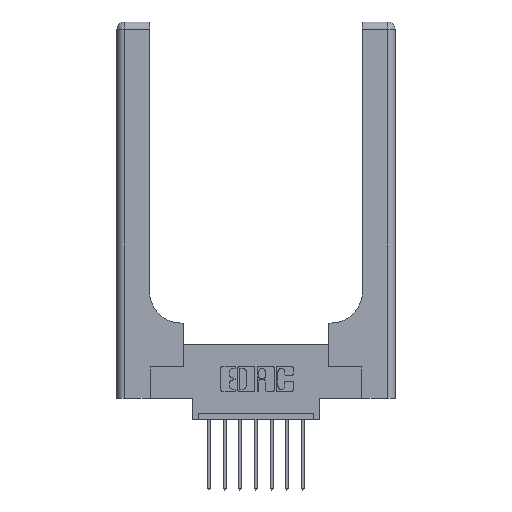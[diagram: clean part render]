
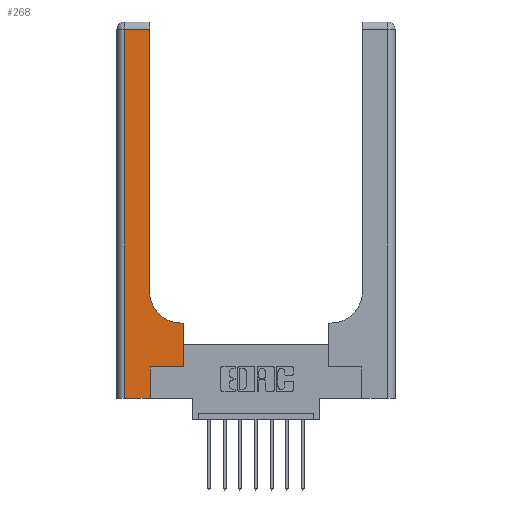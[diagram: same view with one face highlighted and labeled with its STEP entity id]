
A CAD part, top view. The second image highlights one B-rep face of the part: STEP entity #268.
In plain terms, the highlighted planar face has unit normal (0, 0, 1).
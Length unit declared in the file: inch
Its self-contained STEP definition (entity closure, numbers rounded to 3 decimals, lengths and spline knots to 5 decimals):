
#268 = ADVANCED_FACE ( 'NONE', ( #9677 ), #9599, .F. ) ;
#281 = VECTOR ( 'NONE', #3276, 39.37008 ) ;
#473 = EDGE_LOOP ( 'NONE', ( #7348, #3690, #8259, #9559, #8176, #2002, #1999, #13396, #4177 ) ) ;
#953 = LINE ( 'NONE', #8980, #11258 ) ;
#1074 = EDGE_CURVE ( 'NONE', #9855, #10278, #6020, .T. ) ;
#1240 = EDGE_CURVE ( 'NONE', #3831, #9855, #10203, .T. ) ;
#1338 = CARTESIAN_POINT ( 'NONE',  ( 0.528, 0.6, 0.37 ) ) ;
#1574 = LINE ( 'NONE', #5980, #10350 ) ;
#1582 = CARTESIAN_POINT ( 'NONE',  ( 0., 2.94, 0.37 ) ) ;
#1621 = DIRECTION ( 'NONE',  ( 1., 0., 0. ) ) ;
#1999 = ORIENTED_EDGE ( 'NONE', *, *, #14605, .T. ) ;
#2002 = ORIENTED_EDGE ( 'NONE', *, *, #8616, .T. ) ;
#2029 = CARTESIAN_POINT ( 'NONE',  ( 0.26, 0.6, 0.37 ) ) ;
#2476 = CARTESIAN_POINT ( 'NONE',  ( 0.26, 3., 0.37 ) ) ;
#2535 = DIRECTION ( 'NONE',  ( -1., 0., 0. ) ) ;
#2657 = CARTESIAN_POINT ( 'NONE',  ( 0.06, 0., 0.37 ) ) ;
#3129 = DIRECTION ( 'NONE',  ( 1., 0., 0. ) ) ;
#3276 = DIRECTION ( 'NONE',  ( -1., 0., 0. ) ) ;
#3508 = EDGE_CURVE ( 'NONE', #3846, #7573, #11775, .T. ) ;
#3520 = DIRECTION ( 'NONE',  ( 0., 0., -1. ) ) ;
#3690 = ORIENTED_EDGE ( 'NONE', *, *, #3508, .T. ) ;
#3748 = CARTESIAN_POINT ( 'NONE',  ( 0.06, 3., 0.37 ) ) ;
#3753 = VERTEX_POINT ( 'NONE', #8074 ) ;
#3831 = VERTEX_POINT ( 'NONE', #1338 ) ;
#3846 = VERTEX_POINT ( 'NONE', #7935 ) ;
#3858 = VECTOR ( 'NONE', #3129, 39.37008 ) ;
#3957 = CARTESIAN_POINT ( 'NONE',  ( 0., 3., 0.37 ) ) ;
#3981 = LINE ( 'NONE', #8408, #12728 ) ;
#4177 = ORIENTED_EDGE ( 'NONE', *, *, #1074, .T. ) ;
#4865 = LINE ( 'NONE', #2476, #13954 ) ;
#5476 = CARTESIAN_POINT ( 'NONE',  ( 0.265, 0., 0.37 ) ) ;
#5980 = CARTESIAN_POINT ( 'NONE',  ( 0.528, 0.25, 0.37 ) ) ;
#6020 = CIRCLE ( 'NONE', #10579, 0.25 ) ;
#6191 = EDGE_CURVE ( 'NONE', #7573, #10110, #14022, .T. ) ;
#7010 = EDGE_CURVE ( 'NONE', #13799, #3753, #3981, .T. ) ;
#7271 = DIRECTION ( 'NONE',  ( 0., 1., 0. ) ) ;
#7348 = ORIENTED_EDGE ( 'NONE', *, *, #8216, .T. ) ;
#7573 = VERTEX_POINT ( 'NONE', #13841 ) ;
#7856 = LINE ( 'NONE', #8767, #3858 ) ;
#7935 = CARTESIAN_POINT ( 'NONE',  ( 0.26, 2.94, 0.37 ) ) ;
#8074 = CARTESIAN_POINT ( 'NONE',  ( 0.265, 0.25, 0.37 ) ) ;
#8092 = DIRECTION ( 'NONE',  ( 1., 0., 0. ) ) ;
#8176 = ORIENTED_EDGE ( 'NONE', *, *, #7010, .T. ) ;
#8216 = EDGE_CURVE ( 'NONE', #10278, #3846, #4865, .T. ) ;
#8259 = ORIENTED_EDGE ( 'NONE', *, *, #6191, .T. ) ;
#8408 = CARTESIAN_POINT ( 'NONE',  ( 0.265, 0., 0.37 ) ) ;
#8616 = EDGE_CURVE ( 'NONE', #3753, #13579, #7856, .T. ) ;
#8767 = CARTESIAN_POINT ( 'NONE',  ( 0.265, 0.25, 0.37 ) ) ;
#8980 = CARTESIAN_POINT ( 'NONE',  ( 0., 0., 0.37 ) ) ;
#9240 = CARTESIAN_POINT ( 'NONE',  ( 0.51, 0.85, 0.37 ) ) ;
#9559 = ORIENTED_EDGE ( 'NONE', *, *, #10294, .T. ) ;
#9599 = PLANE ( 'NONE',  #14229 ) ;
#9677 = FACE_OUTER_BOUND ( 'NONE', #473, .T. ) ;
#9855 = VERTEX_POINT ( 'NONE', #10279 ) ;
#10110 = VERTEX_POINT ( 'NONE', #2657 ) ;
#10203 = LINE ( 'NONE', #2029, #281 ) ;
#10278 = VERTEX_POINT ( 'NONE', #10400 ) ;
#10279 = CARTESIAN_POINT ( 'NONE',  ( 0.51, 0.6, 0.37 ) ) ;
#10294 = EDGE_CURVE ( 'NONE', #10110, #13799, #953, .T. ) ;
#10350 = VECTOR ( 'NONE', #7271, 39.37008 ) ;
#10400 = CARTESIAN_POINT ( 'NONE',  ( 0.26, 0.85, 0.37 ) ) ;
#10579 = AXIS2_PLACEMENT_3D ( 'NONE', #9240, #3520, #8092 ) ;
#10660 = DIRECTION ( 'NONE',  ( -1., 0., 0. ) ) ;
#10769 = VECTOR ( 'NONE', #10660, 39.37008 ) ;
#11258 = VECTOR ( 'NONE', #1621, 39.37008 ) ;
#11775 = LINE ( 'NONE', #1582, #10769 ) ;
#11856 = DIRECTION ( 'NONE',  ( 0., 1., 0. ) ) ;
#12728 = VECTOR ( 'NONE', #11856, 39.37008 ) ;
#12757 = CARTESIAN_POINT ( 'NONE',  ( 0.528, 0.25, 0.37 ) ) ;
#12887 = DIRECTION ( 'NONE',  ( 0., 1., 0. ) ) ;
#12899 = DIRECTION ( 'NONE',  ( 0., -1., 0. ) ) ;
#13396 = ORIENTED_EDGE ( 'NONE', *, *, #1240, .T. ) ;
#13579 = VERTEX_POINT ( 'NONE', #12757 ) ;
#13799 = VERTEX_POINT ( 'NONE', #5476 ) ;
#13841 = CARTESIAN_POINT ( 'NONE',  ( 0.06, 2.94, 0.37 ) ) ;
#13877 = VECTOR ( 'NONE', #12899, 39.37008 ) ;
#13954 = VECTOR ( 'NONE', #12887, 39.37008 ) ;
#14001 = DIRECTION ( 'NONE',  ( 0., 0., -1. ) ) ;
#14022 = LINE ( 'NONE', #3748, #13877 ) ;
#14229 = AXIS2_PLACEMENT_3D ( 'NONE', #3957, #14001, #2535 ) ;
#14605 = EDGE_CURVE ( 'NONE', #13579, #3831, #1574, .T. ) ;
